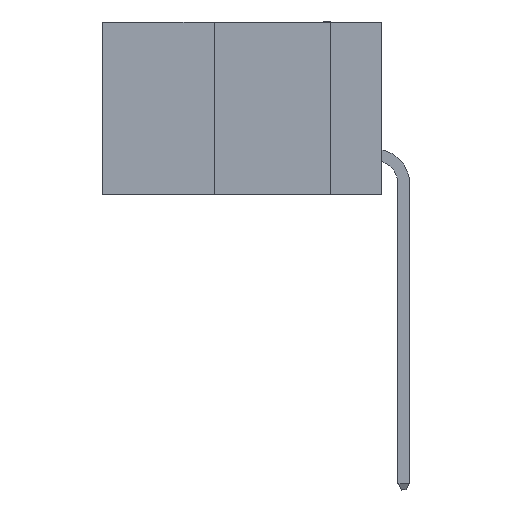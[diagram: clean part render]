
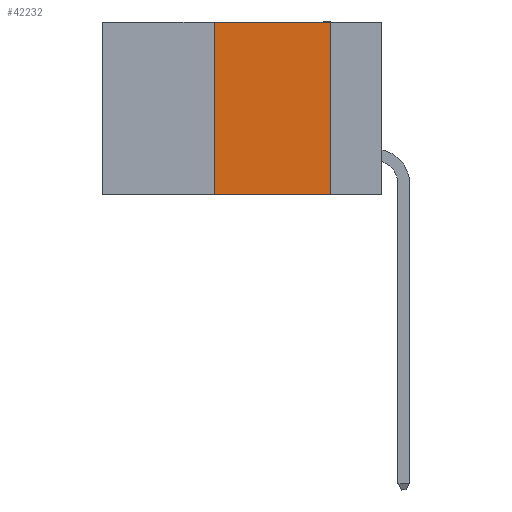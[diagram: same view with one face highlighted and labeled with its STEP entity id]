
A CAD part, left-side view. The second image highlights one B-rep face of the part: STEP entity #42232.
In plain terms, the highlighted planar face has unit normal (-1, 0, 0).
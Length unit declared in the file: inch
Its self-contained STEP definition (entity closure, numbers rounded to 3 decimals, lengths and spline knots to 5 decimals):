
#2008 = DIRECTION ( 'NONE',  ( 0., 0., -1. ) ) ;
#3056 = ORIENTED_EDGE ( 'NONE', *, *, #5257, .F. ) ;
#3158 = VECTOR ( 'NONE', #5083, 39.37008 ) ;
#3900 = FACE_OUTER_BOUND ( 'NONE', #43449, .T. ) ;
#4502 = VERTEX_POINT ( 'NONE', #36841 ) ;
#4827 = EDGE_CURVE ( 'NONE', #17104, #9637, #13695, .T. ) ;
#5083 = DIRECTION ( 'NONE',  ( 0., 0., 1. ) ) ;
#5114 = CARTESIAN_POINT ( 'NONE',  ( 0., 0.6, -0.37 ) ) ;
#5257 = EDGE_CURVE ( 'NONE', #4502, #17104, #11045, .T. ) ;
#5654 = DIRECTION ( 'NONE',  ( 0., -1., 0. ) ) ;
#7309 = DIRECTION ( 'NONE',  ( 0., 0., -1. ) ) ;
#8316 = CARTESIAN_POINT ( 'NONE',  ( 0., 0.36, 0. ) ) ;
#9637 = VERTEX_POINT ( 'NONE', #41325 ) ;
#10544 = VECTOR ( 'NONE', #5654, 39.37008 ) ;
#11021 = EDGE_CURVE ( 'NONE', #9637, #37123, #14351, .T. ) ;
#11045 = LINE ( 'NONE', #8316, #3158 ) ;
#13695 = LINE ( 'NONE', #22095, #10544 ) ;
#14351 = LINE ( 'NONE', #20408, #28014 ) ;
#17104 = VERTEX_POINT ( 'NONE', #19461 ) ;
#17471 = ORIENTED_EDGE ( 'NONE', *, *, #4827, .F. ) ;
#18602 = ORIENTED_EDGE ( 'NONE', *, *, #35047, .T. ) ;
#19461 = CARTESIAN_POINT ( 'NONE',  ( 0., 0.36, 0. ) ) ;
#20408 = CARTESIAN_POINT ( 'NONE',  ( 0., 0.11, 0. ) ) ;
#20441 = CARTESIAN_POINT ( 'NONE',  ( 0., 0.11, -0.37 ) ) ;
#21534 = LINE ( 'NONE', #5114, #29465 ) ;
#22095 = CARTESIAN_POINT ( 'NONE',  ( 0., 0.6, 0. ) ) ;
#25972 = DIRECTION ( 'NONE',  ( 1., 0., 0. ) ) ;
#28014 = VECTOR ( 'NONE', #7309, 39.37008 ) ;
#29465 = VECTOR ( 'NONE', #39674, 39.37008 ) ;
#29514 = PLANE ( 'NONE',  #33303 ) ;
#33303 = AXIS2_PLACEMENT_3D ( 'NONE', #42602, #25972, #2008 ) ;
#35040 = ORIENTED_EDGE ( 'NONE', *, *, #11021, .F. ) ;
#35047 = EDGE_CURVE ( 'NONE', #4502, #37123, #21534, .T. ) ;
#36841 = CARTESIAN_POINT ( 'NONE',  ( 0., 0.36, -0.37 ) ) ;
#37123 = VERTEX_POINT ( 'NONE', #20441 ) ;
#39674 = DIRECTION ( 'NONE',  ( 0., -1., 0. ) ) ;
#41325 = CARTESIAN_POINT ( 'NONE',  ( 0., 0.11, 0. ) ) ;
#42232 = ADVANCED_FACE ( 'NONE', ( #3900 ), #29514, .F. ) ;
#42602 = CARTESIAN_POINT ( 'NONE',  ( 0., 0.6, 0. ) ) ;
#43449 = EDGE_LOOP ( 'NONE', ( #35040, #17471, #3056, #18602 ) ) ;
